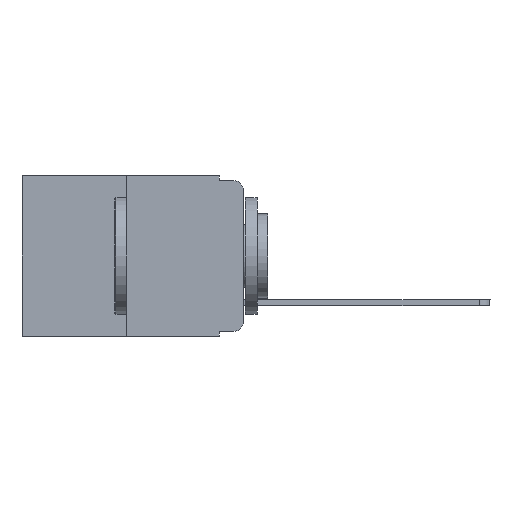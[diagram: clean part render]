
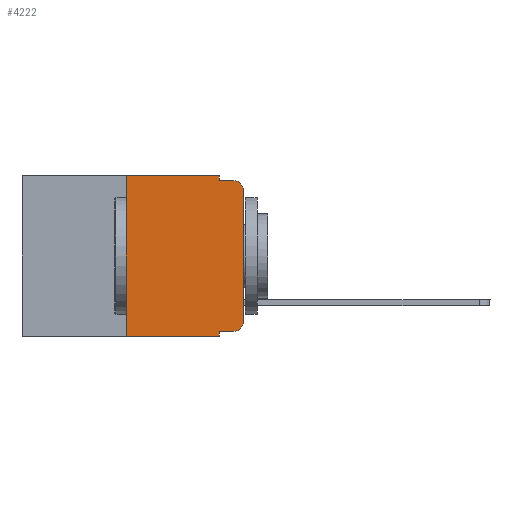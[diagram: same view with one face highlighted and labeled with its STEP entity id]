
A CAD part, left-side view. The second image highlights one B-rep face of the part: STEP entity #4222.
In plain terms, the highlighted planar face has unit normal (-1, 0, 0).
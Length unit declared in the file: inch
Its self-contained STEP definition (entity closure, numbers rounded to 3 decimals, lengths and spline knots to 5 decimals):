
#102 = EDGE_CURVE ( 'NONE', #13862, #10988, #3428, .T. ) ;
#159 = DIRECTION ( 'NONE',  ( -1., 0., 0. ) ) ;
#513 = LINE ( 'NONE', #676, #6074 ) ;
#676 = CARTESIAN_POINT ( 'NONE',  ( 0., 0.473, 0. ) ) ;
#753 = CARTESIAN_POINT ( 'NONE',  ( 0., 0.473, -0.343 ) ) ;
#871 = EDGE_CURVE ( 'NONE', #14006, #15225, #12369, .T. ) ;
#894 = CARTESIAN_POINT ( 'NONE',  ( 0., 0.02, -0.01 ) ) ;
#1057 = CIRCLE ( 'NONE', #10372, 0.02 ) ;
#1276 = VERTEX_POINT ( 'NONE', #10574 ) ;
#1861 = ORIENTED_EDGE ( 'NONE', *, *, #7715, .T. ) ;
#2130 = EDGE_CURVE ( 'NONE', #16152, #15460, #9207, .T. ) ;
#2612 = ORIENTED_EDGE ( 'NONE', *, *, #2130, .F. ) ;
#2784 = EDGE_LOOP ( 'NONE', ( #1861, #14809, #16418, #14395, #10962, #9097, #10101, #2612, #7064, #8353 ) ) ;
#3110 = DIRECTION ( 'NONE',  ( 0., -1., 0. ) ) ;
#3319 = EDGE_CURVE ( 'NONE', #11106, #8091, #13515, .T. ) ;
#3428 = LINE ( 'NONE', #15114, #13563 ) ;
#3758 = DIRECTION ( 'NONE',  ( 0., 0., 1. ) ) ;
#3994 = VECTOR ( 'NONE', #4376, 39.37008 ) ;
#4222 = ADVANCED_FACE ( 'NONE', ( #6595 ), #5182, .F. ) ;
#4278 = EDGE_CURVE ( 'NONE', #15225, #1276, #513, .T. ) ;
#4376 = DIRECTION ( 'NONE',  ( 0., 0., -1. ) ) ;
#4760 = CARTESIAN_POINT ( 'NONE',  ( 0., 0.25, 0. ) ) ;
#4841 = LINE ( 'NONE', #15285, #10506 ) ;
#5182 = PLANE ( 'NONE',  #5812 ) ;
#5586 = LINE ( 'NONE', #753, #11039 ) ;
#5812 = AXIS2_PLACEMENT_3D ( 'NONE', #6516, #9248, #15380 ) ;
#6074 = VECTOR ( 'NONE', #3110, 39.37008 ) ;
#6314 = CARTESIAN_POINT ( 'NONE',  ( 0., 0.02, -0.333 ) ) ;
#6335 = DIRECTION ( 'NONE',  ( 0., -1., 0. ) ) ;
#6378 = DIRECTION ( 'NONE',  ( 0., 0., -1. ) ) ;
#6492 = CARTESIAN_POINT ( 'NONE',  ( 0., 0.02, -0.313 ) ) ;
#6516 = CARTESIAN_POINT ( 'NONE',  ( 0., 0.473, 0. ) ) ;
#6595 = FACE_OUTER_BOUND ( 'NONE', #2784, .T. ) ;
#6830 = EDGE_CURVE ( 'NONE', #1276, #13862, #10608, .T. ) ;
#7064 = ORIENTED_EDGE ( 'NONE', *, *, #13468, .T. ) ;
#7715 = EDGE_CURVE ( 'NONE', #8091, #14840, #8820, .T. ) ;
#8091 = VERTEX_POINT ( 'NONE', #12833 ) ;
#8353 = ORIENTED_EDGE ( 'NONE', *, *, #3319, .T. ) ;
#8420 = VECTOR ( 'NONE', #8424, 39.37008 ) ;
#8424 = DIRECTION ( 'NONE',  ( 0., 0., 1. ) ) ;
#8788 = VECTOR ( 'NONE', #11634, 39.37008 ) ;
#8820 = LINE ( 'NONE', #14266, #12007 ) ;
#8931 = CARTESIAN_POINT ( 'NONE',  ( 0., 0., -0.03 ) ) ;
#9097 = ORIENTED_EDGE ( 'NONE', *, *, #871, .F. ) ;
#9148 = CARTESIAN_POINT ( 'NONE',  ( 0., 0.25, 0. ) ) ;
#9207 = LINE ( 'NONE', #15415, #8788 ) ;
#9212 = CARTESIAN_POINT ( 'NONE',  ( 0., 0.25, -0.343 ) ) ;
#9248 = DIRECTION ( 'NONE',  ( 1., 0., 0. ) ) ;
#10101 = ORIENTED_EDGE ( 'NONE', *, *, #11936, .T. ) ;
#10372 = AXIS2_PLACEMENT_3D ( 'NONE', #11622, #15498, #6378 ) ;
#10402 = DIRECTION ( 'NONE',  ( 0., 0., -1. ) ) ;
#10506 = VECTOR ( 'NONE', #6335, 39.37008 ) ;
#10574 = CARTESIAN_POINT ( 'NONE',  ( 0., 0.051, 0. ) ) ;
#10608 = LINE ( 'NONE', #14407, #3994 ) ;
#10832 = CARTESIAN_POINT ( 'NONE',  ( 0., 0.051, -0.333 ) ) ;
#10962 = ORIENTED_EDGE ( 'NONE', *, *, #4278, .F. ) ;
#10988 = VERTEX_POINT ( 'NONE', #894 ) ;
#11039 = VECTOR ( 'NONE', #12360, 39.37008 ) ;
#11106 = VERTEX_POINT ( 'NONE', #6314 ) ;
#11237 = DIRECTION ( 'NONE',  ( 0., -1., 0. ) ) ;
#11455 = CARTESIAN_POINT ( 'NONE',  ( 0., 0.051, -0.343 ) ) ;
#11622 = CARTESIAN_POINT ( 'NONE',  ( 0., 0.02, -0.03 ) ) ;
#11634 = DIRECTION ( 'NONE',  ( 0., 0., -1. ) ) ;
#11936 = EDGE_CURVE ( 'NONE', #14006, #15460, #5586, .T. ) ;
#12007 = VECTOR ( 'NONE', #3758, 39.37008 ) ;
#12360 = DIRECTION ( 'NONE',  ( 0., -1., 0. ) ) ;
#12369 = LINE ( 'NONE', #4760, #8420 ) ;
#12833 = CARTESIAN_POINT ( 'NONE',  ( 0., 0., -0.313 ) ) ;
#13468 = EDGE_CURVE ( 'NONE', #16152, #11106, #4841, .T. ) ;
#13515 = CIRCLE ( 'NONE', #15419, 0.02 ) ;
#13563 = VECTOR ( 'NONE', #11237, 39.37008 ) ;
#13853 = CARTESIAN_POINT ( 'NONE',  ( 0., 0.051, -0.01 ) ) ;
#13862 = VERTEX_POINT ( 'NONE', #13853 ) ;
#14006 = VERTEX_POINT ( 'NONE', #9212 ) ;
#14266 = CARTESIAN_POINT ( 'NONE',  ( 0., 0., 0. ) ) ;
#14395 = ORIENTED_EDGE ( 'NONE', *, *, #6830, .F. ) ;
#14407 = CARTESIAN_POINT ( 'NONE',  ( 0., 0.051, 0. ) ) ;
#14809 = ORIENTED_EDGE ( 'NONE', *, *, #15511, .T. ) ;
#14840 = VERTEX_POINT ( 'NONE', #8931 ) ;
#15114 = CARTESIAN_POINT ( 'NONE',  ( 0., 0.051, -0.01 ) ) ;
#15225 = VERTEX_POINT ( 'NONE', #9148 ) ;
#15285 = CARTESIAN_POINT ( 'NONE',  ( 0., 0.051, -0.333 ) ) ;
#15380 = DIRECTION ( 'NONE',  ( 0., 0., -1. ) ) ;
#15415 = CARTESIAN_POINT ( 'NONE',  ( 0., 0.051, 0. ) ) ;
#15419 = AXIS2_PLACEMENT_3D ( 'NONE', #6492, #159, #10402 ) ;
#15460 = VERTEX_POINT ( 'NONE', #11455 ) ;
#15498 = DIRECTION ( 'NONE',  ( -1., 0., 0. ) ) ;
#15511 = EDGE_CURVE ( 'NONE', #14840, #10988, #1057, .T. ) ;
#16152 = VERTEX_POINT ( 'NONE', #10832 ) ;
#16418 = ORIENTED_EDGE ( 'NONE', *, *, #102, .F. ) ;
